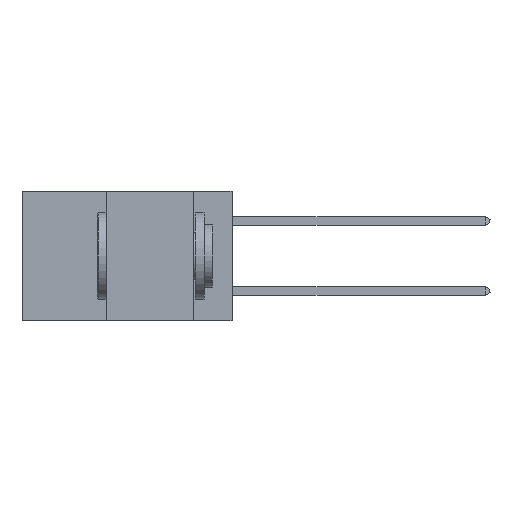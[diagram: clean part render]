
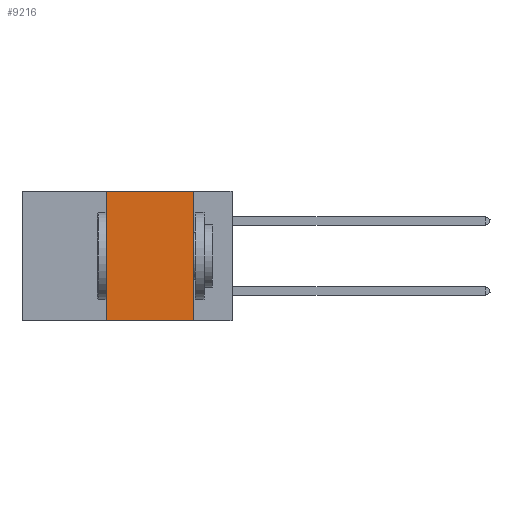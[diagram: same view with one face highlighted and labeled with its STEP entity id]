
A CAD part, left-side view. The second image highlights one B-rep face of the part: STEP entity #9216.
In plain terms, the highlighted planar face has unit normal (-1, 0, 0).
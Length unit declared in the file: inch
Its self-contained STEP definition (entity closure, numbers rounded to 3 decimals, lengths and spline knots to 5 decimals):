
#70 = CARTESIAN_POINT ( 'NONE',  ( 0., 0.11, -0.37 ) ) ;
#528 = FACE_OUTER_BOUND ( 'NONE', #26709, .T. ) ;
#2334 = LINE ( 'NONE', #11979, #30370 ) ;
#3489 = DIRECTION ( 'NONE',  ( 0., -1., 0. ) ) ;
#5266 = ORIENTED_EDGE ( 'NONE', *, *, #28268, .F. ) ;
#6397 = EDGE_CURVE ( 'NONE', #7135, #16389, #14077, .T. ) ;
#6787 = DIRECTION ( 'NONE',  ( 0., 0., 1. ) ) ;
#7135 = VERTEX_POINT ( 'NONE', #13143 ) ;
#7876 = CARTESIAN_POINT ( 'NONE',  ( 0., 0.6, 0. ) ) ;
#8806 = PLANE ( 'NONE',  #21118 ) ;
#9216 = ADVANCED_FACE ( 'NONE', ( #528 ), #8806, .F. ) ;
#11425 = DIRECTION ( 'NONE',  ( 0., 0., -1. ) ) ;
#11473 = DIRECTION ( 'NONE',  ( 0., 0., -1. ) ) ;
#11979 = CARTESIAN_POINT ( 'NONE',  ( 0., 0.36, 0. ) ) ;
#12810 = VERTEX_POINT ( 'NONE', #70 ) ;
#13040 = ORIENTED_EDGE ( 'NONE', *, *, #29305, .T. ) ;
#13143 = CARTESIAN_POINT ( 'NONE',  ( 0., 0.36, 0. ) ) ;
#13412 = DIRECTION ( 'NONE',  ( 0., -1., 0. ) ) ;
#14077 = LINE ( 'NONE', #7876, #34352 ) ;
#16389 = VERTEX_POINT ( 'NONE', #18807 ) ;
#17213 = CARTESIAN_POINT ( 'NONE',  ( 0., 0.6, 0. ) ) ;
#17315 = CARTESIAN_POINT ( 'NONE',  ( 0., 0.6, -0.37 ) ) ;
#18807 = CARTESIAN_POINT ( 'NONE',  ( 0., 0.11, 0. ) ) ;
#20864 = EDGE_CURVE ( 'NONE', #22537, #7135, #2334, .T. ) ;
#21118 = AXIS2_PLACEMENT_3D ( 'NONE', #17213, #25091, #11473 ) ;
#21742 = VECTOR ( 'NONE', #3489, 39.37008 ) ;
#22537 = VERTEX_POINT ( 'NONE', #30889 ) ;
#24298 = ORIENTED_EDGE ( 'NONE', *, *, #6397, .F. ) ;
#25091 = DIRECTION ( 'NONE',  ( 1., 0., 0. ) ) ;
#25133 = ORIENTED_EDGE ( 'NONE', *, *, #20864, .F. ) ;
#26063 = LINE ( 'NONE', #17315, #21742 ) ;
#26709 = EDGE_LOOP ( 'NONE', ( #5266, #24298, #25133, #13040 ) ) ;
#27069 = VECTOR ( 'NONE', #11425, 39.37008 ) ;
#28268 = EDGE_CURVE ( 'NONE', #16389, #12810, #34424, .T. ) ;
#29305 = EDGE_CURVE ( 'NONE', #22537, #12810, #26063, .T. ) ;
#30370 = VECTOR ( 'NONE', #6787, 39.37008 ) ;
#30889 = CARTESIAN_POINT ( 'NONE',  ( 0., 0.36, -0.37 ) ) ;
#32530 = CARTESIAN_POINT ( 'NONE',  ( 0., 0.11, 0. ) ) ;
#34352 = VECTOR ( 'NONE', #13412, 39.37008 ) ;
#34424 = LINE ( 'NONE', #32530, #27069 ) ;
